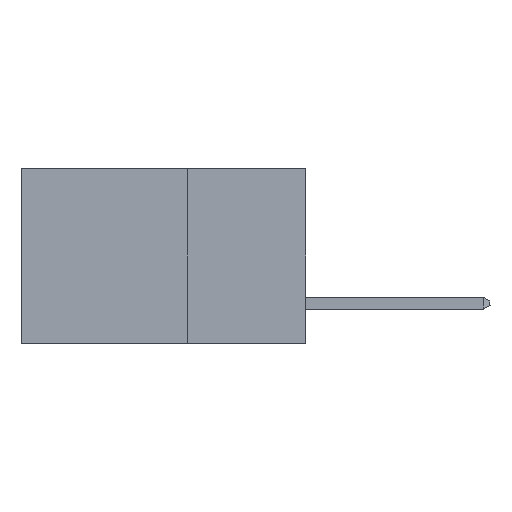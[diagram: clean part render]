
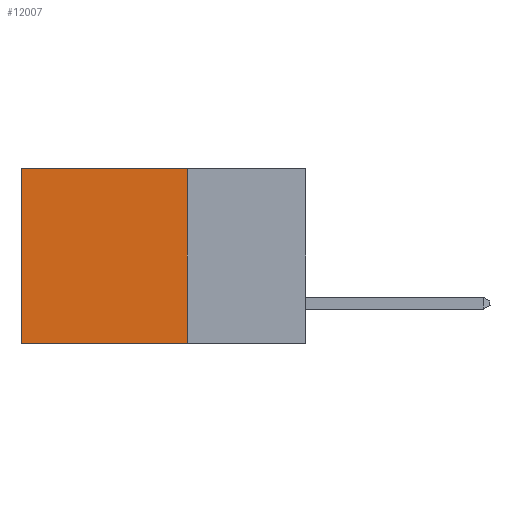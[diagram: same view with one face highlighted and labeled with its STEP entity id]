
A CAD part, left-side view. The second image highlights one B-rep face of the part: STEP entity #12007.
In plain terms, the highlighted planar face has unit normal (-1, 0, 0).
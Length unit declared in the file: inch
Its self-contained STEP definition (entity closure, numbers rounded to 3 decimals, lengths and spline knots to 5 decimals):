
#323 = PLANE ( 'NONE',  #14841 ) ;
#983 = CARTESIAN_POINT ( 'NONE',  ( 0.298, 0.6, -0.37 ) ) ;
#1729 = VERTEX_POINT ( 'NONE', #4714 ) ;
#4280 = ORIENTED_EDGE ( 'NONE', *, *, #9969, .F. ) ;
#4714 = CARTESIAN_POINT ( 'NONE',  ( 0.298, 0.25, -0.37 ) ) ;
#4903 = CARTESIAN_POINT ( 'NONE',  ( 0.298, 0.25, 0. ) ) ;
#5517 = EDGE_LOOP ( 'NONE', ( #20471, #4280, #18326, #14861 ) ) ;
#6333 = LINE ( 'NONE', #20232, #11384 ) ;
#7296 = CARTESIAN_POINT ( 'NONE',  ( 0.298, 0.25, 0. ) ) ;
#7399 = DIRECTION ( 'NONE',  ( 0., 1., 0. ) ) ;
#7450 = EDGE_CURVE ( 'NONE', #18560, #11516, #16765, .T. ) ;
#8181 = CARTESIAN_POINT ( 'NONE',  ( 0.298, 0.6, 0. ) ) ;
#8878 = CARTESIAN_POINT ( 'NONE',  ( 0.298, 0.25, 0. ) ) ;
#9969 = EDGE_CURVE ( 'NONE', #1729, #20621, #11044, .T. ) ;
#10489 = VECTOR ( 'NONE', #7399, 39.37008 ) ;
#10520 = DIRECTION ( 'NONE',  ( 0., 1., 0. ) ) ;
#11044 = LINE ( 'NONE', #12075, #18290 ) ;
#11313 = EDGE_CURVE ( 'NONE', #11516, #20621, #6333, .T. ) ;
#11384 = VECTOR ( 'NONE', #17311, 39.37008 ) ;
#11516 = VERTEX_POINT ( 'NONE', #8181 ) ;
#12007 = ADVANCED_FACE ( 'NONE', ( #16669 ), #323, .F. ) ;
#12053 = CARTESIAN_POINT ( 'NONE',  ( 0.298, 0.25, 0. ) ) ;
#12075 = CARTESIAN_POINT ( 'NONE',  ( 0.298, 0.25, -0.37 ) ) ;
#14841 = AXIS2_PLACEMENT_3D ( 'NONE', #4903, #16151, #18044 ) ;
#14861 = ORIENTED_EDGE ( 'NONE', *, *, #7450, .T. ) ;
#15866 = EDGE_CURVE ( 'NONE', #18560, #1729, #20699, .T. ) ;
#16151 = DIRECTION ( 'NONE',  ( 1., 0., 0. ) ) ;
#16669 = FACE_OUTER_BOUND ( 'NONE', #5517, .T. ) ;
#16714 = VECTOR ( 'NONE', #16920, 39.37008 ) ;
#16765 = LINE ( 'NONE', #8878, #10489 ) ;
#16920 = DIRECTION ( 'NONE',  ( 0., 0., -1. ) ) ;
#17311 = DIRECTION ( 'NONE',  ( 0., 0., -1. ) ) ;
#18044 = DIRECTION ( 'NONE',  ( 0., 0., -1. ) ) ;
#18290 = VECTOR ( 'NONE', #10520, 39.37008 ) ;
#18326 = ORIENTED_EDGE ( 'NONE', *, *, #15866, .F. ) ;
#18560 = VERTEX_POINT ( 'NONE', #12053 ) ;
#20232 = CARTESIAN_POINT ( 'NONE',  ( 0.298, 0.6, 0. ) ) ;
#20471 = ORIENTED_EDGE ( 'NONE', *, *, #11313, .T. ) ;
#20621 = VERTEX_POINT ( 'NONE', #983 ) ;
#20699 = LINE ( 'NONE', #7296, #16714 ) ;
